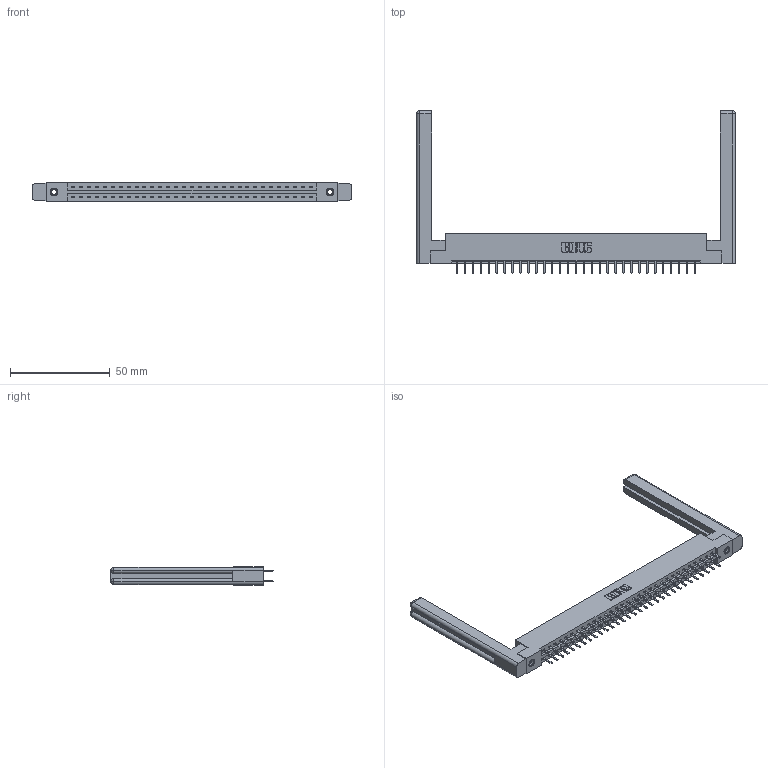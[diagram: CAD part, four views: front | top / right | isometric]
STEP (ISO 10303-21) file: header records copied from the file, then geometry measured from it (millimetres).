
FILE_DESCRIPTION (( 'STEP AP203' ), '1' );
FILE_NAME ('337-062-520-258.STEP', '2019-10-09T21:04:20', ( '' ), ( '' ), 'SwSTEP 2.0', 'SolidWorks 2016', '' );
FILE_SCHEMA (( 'CONFIG_CONTROL_DESIGN' ));
Length unit declared in the file: inch
Products named in the file (5): 307-220-058; 345-250-001_345-250-001-102; 345-292-001_345-293-120; 337 Part_Flush Mounting Lugs - 0.156 Dia-TI; 337-062-520-258
Assembly tree (67 placements, depth 2):
  337-062-520-258
    337 Part_Flush Mounting Lugs - 0.156 Dia-TI
    345-292-001_345-293-120  x62
    345-250-001_345-250-001-102  x2
    307-220-058  x2
Bounding box: 159.46 x 81.11 x 9.4 mm (x, y, z)
Volume: 23774 mm3; surface area: 23664.2 mm2
Topology: 67 solids, 67 shells, 3852 faces, 11143 edges, 7250 vertices
Faces by surface type: plane 2634, cylinder 1194, cone 12, torus 12
Entity records: 28206 total; most frequent: CARTESIAN_POINT 4781, ORIENTED_EDGE 4644, DIRECTION 4090, EDGE_CURVE 2322, VECTOR 2142, LINE 2142, VERTEX_POINT 1538, AXIS2_PLACEMENT_3D 974
